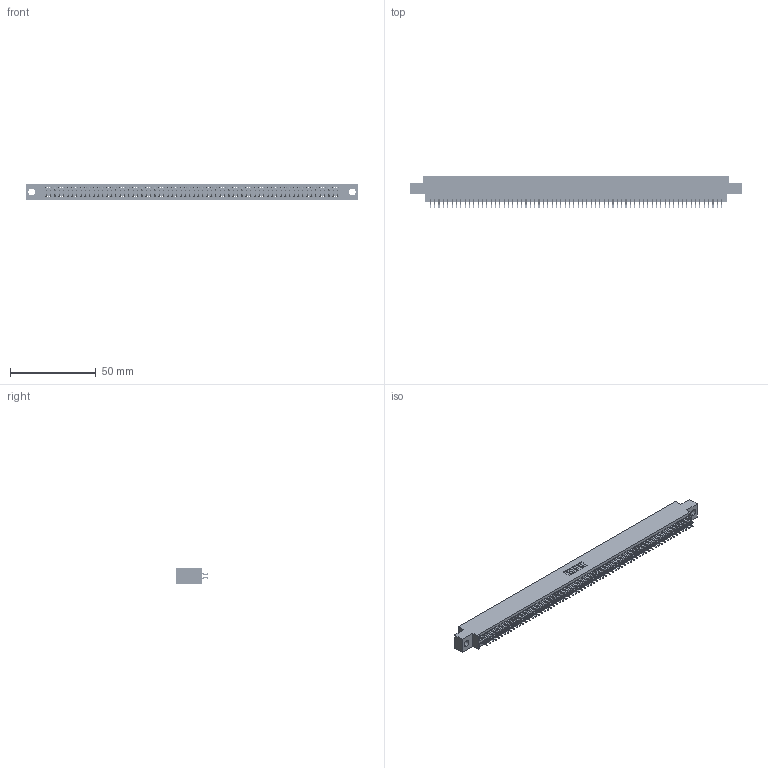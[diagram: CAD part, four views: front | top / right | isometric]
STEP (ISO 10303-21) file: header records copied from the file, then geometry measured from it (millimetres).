
FILE_DESCRIPTION (( 'STEP AP203' ), '1' );
FILE_NAME ('395-136-556-804.STEP', '2021-06-18T03:02:45', ( '' ), ( '' ), 'SwSTEP 2.0', 'SolidWorks 2020', '' );
FILE_SCHEMA (( 'CONFIG_CONTROL_DESIGN' ));
Length unit declared in the file: inch
Products named in the file (3): 345-292-001_556 Tail; 345 Part_0.170 Offset - 0.156 Dia-TI; 395-136-556-804
Assembly tree (137 placements, depth 2):
  395-136-556-804
    345 Part_0.170 Offset - 0.156 Dia-TI
    345-292-001_556 Tail  x136
Bounding box: 193.93 x 19.24 x 9.4 mm (x, y, z)
Volume: 18855.1 mm3; surface area: 28250.6 mm2
Topology: 137 solids, 137 shells, 7760 faces, 23101 edges, 15218 vertices
Faces by surface type: plane 5130, cylinder 2630
Entity records: 50625 total; most frequent: CARTESIAN_POINT 8482, ORIENTED_EDGE 8402, DIRECTION 7433, EDGE_CURVE 4201, VECTOR 3789, LINE 3789, VERTEX_POINT 2798, AXIS2_PLACEMENT_3D 1822
